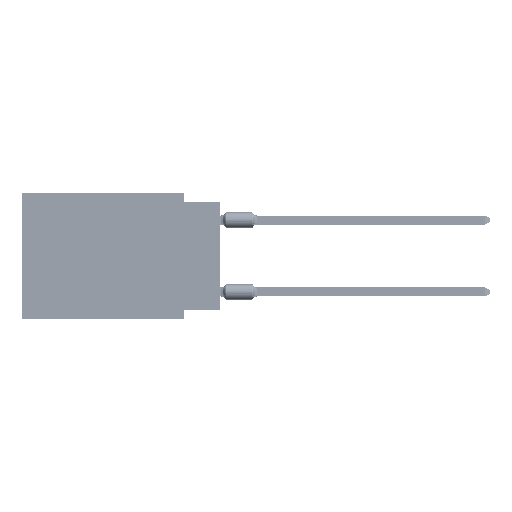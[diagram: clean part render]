
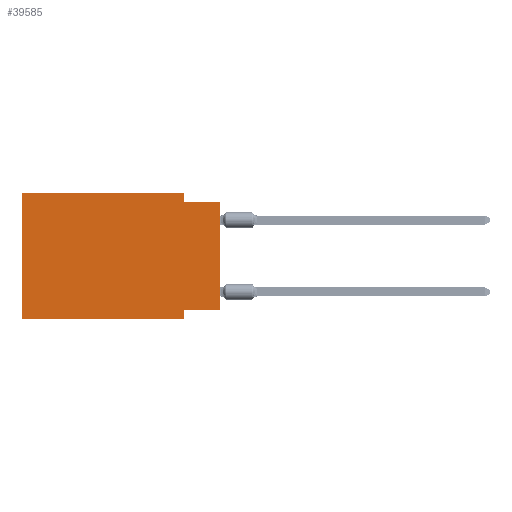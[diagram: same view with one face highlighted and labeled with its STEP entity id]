
A CAD part, left-side view. The second image highlights one B-rep face of the part: STEP entity #39585.
In plain terms, the highlighted planar face has unit normal (-1, 0, 0).
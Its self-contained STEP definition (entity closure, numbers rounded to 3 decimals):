
#471 = DIRECTION ( 'NONE',  ( 0., 0., -1. ) ) ;
#1553 = CARTESIAN_POINT ( 'NONE',  ( 0., 2.54, -8.255 ) ) ;
#2929 = EDGE_CURVE ( 'NONE', #44867, #82245, #107973, .T. ) ;
#6855 = LINE ( 'NONE', #51619, #43637 ) ;
#7664 = CARTESIAN_POINT ( 'NONE',  ( 0., 13.97, -8.89 ) ) ;
#10004 = VECTOR ( 'NONE', #471, 1000. ) ;
#10639 = DIRECTION ( 'NONE',  ( 0., 0., -1. ) ) ;
#10737 = EDGE_LOOP ( 'NONE', ( #77970, #42111, #17066, #55393, #105549, #76136, #22243, #19963 ) ) ;
#13198 = EDGE_CURVE ( 'NONE', #44867, #31810, #33668, .T. ) ;
#14741 = VECTOR ( 'NONE', #26188, 1000. ) ;
#14808 = VERTEX_POINT ( 'NONE', #32982 ) ;
#16562 = EDGE_CURVE ( 'NONE', #79509, #60646, #83438, .T. ) ;
#17066 = ORIENTED_EDGE ( 'NONE', *, *, #102104, .F. ) ;
#19963 = ORIENTED_EDGE ( 'NONE', *, *, #13198, .F. ) ;
#22243 = ORIENTED_EDGE ( 'NONE', *, *, #87698, .F. ) ;
#26188 = DIRECTION ( 'NONE',  ( 0., -1., 0. ) ) ;
#30516 = VECTOR ( 'NONE', #43050, 1000. ) ;
#31810 = VERTEX_POINT ( 'NONE', #1553 ) ;
#32205 = CARTESIAN_POINT ( 'NONE',  ( 0., 0., 0. ) ) ;
#32610 = VERTEX_POINT ( 'NONE', #76518 ) ;
#32982 = CARTESIAN_POINT ( 'NONE',  ( 0., 13.97, 0. ) ) ;
#33668 = LINE ( 'NONE', #85099, #30516 ) ;
#39585 = ADVANCED_FACE ( 'NONE', ( #55048 ), #72182, .F. ) ;
#41398 = DIRECTION ( 'NONE',  ( 0., -1., 0. ) ) ;
#42111 = ORIENTED_EDGE ( 'NONE', *, *, #86768, .F. ) ;
#43050 = DIRECTION ( 'NONE',  ( 0., 1., 0. ) ) ;
#43575 = CARTESIAN_POINT ( 'NONE',  ( 0., 2.54, -8.89 ) ) ;
#43637 = VECTOR ( 'NONE', #84829, 1000. ) ;
#44867 = VERTEX_POINT ( 'NONE', #65329 ) ;
#51619 = CARTESIAN_POINT ( 'NONE',  ( 0., 0., -0.635 ) ) ;
#54789 = VERTEX_POINT ( 'NONE', #64072 ) ;
#55048 = FACE_OUTER_BOUND ( 'NONE', #10737, .T. ) ;
#55305 = VECTOR ( 'NONE', #57617, 1000. ) ;
#55393 = ORIENTED_EDGE ( 'NONE', *, *, #65515, .F. ) ;
#57617 = DIRECTION ( 'NONE',  ( 0., 0., 1. ) ) ;
#60206 = LINE ( 'NONE', #43575, #10004 ) ;
#60646 = VERTEX_POINT ( 'NONE', #80372 ) ;
#60956 = LINE ( 'NONE', #86405, #72630 ) ;
#62259 = DIRECTION ( 'NONE',  ( 1., 0., 0. ) ) ;
#63890 = CARTESIAN_POINT ( 'NONE',  ( 0., 13.97, 0. ) ) ;
#64072 = CARTESIAN_POINT ( 'NONE',  ( 0., 2.54, 0. ) ) ;
#65329 = CARTESIAN_POINT ( 'NONE',  ( 0., 0., -8.255 ) ) ;
#65515 = EDGE_CURVE ( 'NONE', #14808, #54789, #86453, .T. ) ;
#67099 = VECTOR ( 'NONE', #104514, 1000. ) ;
#72182 = PLANE ( 'NONE',  #108007 ) ;
#72630 = VECTOR ( 'NONE', #10639, 1000. ) ;
#76136 = ORIENTED_EDGE ( 'NONE', *, *, #16562, .T. ) ;
#76518 = CARTESIAN_POINT ( 'NONE',  ( 0., 2.54, -0.635 ) ) ;
#77970 = ORIENTED_EDGE ( 'NONE', *, *, #2929, .T. ) ;
#79509 = VERTEX_POINT ( 'NONE', #90200 ) ;
#80372 = CARTESIAN_POINT ( 'NONE',  ( 0., 2.54, -8.89 ) ) ;
#82245 = VERTEX_POINT ( 'NONE', #107384 ) ;
#83438 = LINE ( 'NONE', #7664, #91496 ) ;
#84829 = DIRECTION ( 'NONE',  ( 0., -1., 0. ) ) ;
#85099 = CARTESIAN_POINT ( 'NONE',  ( 0., 0., -8.255 ) ) ;
#85898 = CARTESIAN_POINT ( 'NONE',  ( 0., 13.97, 0. ) ) ;
#86405 = CARTESIAN_POINT ( 'NONE',  ( 0., 2.54, 0. ) ) ;
#86453 = LINE ( 'NONE', #85898, #14741 ) ;
#86768 = EDGE_CURVE ( 'NONE', #32610, #82245, #6855, .T. ) ;
#87698 = EDGE_CURVE ( 'NONE', #31810, #60646, #60206, .T. ) ;
#89306 = DIRECTION ( 'NONE',  ( 0., 0., -1. ) ) ;
#90200 = CARTESIAN_POINT ( 'NONE',  ( 0., 13.97, -8.89 ) ) ;
#91496 = VECTOR ( 'NONE', #41398, 1000. ) ;
#95670 = LINE ( 'NONE', #102313, #67099 ) ;
#102104 = EDGE_CURVE ( 'NONE', #54789, #32610, #60956, .T. ) ;
#102313 = CARTESIAN_POINT ( 'NONE',  ( 0., 13.97, 0. ) ) ;
#102429 = EDGE_CURVE ( 'NONE', #79509, #14808, #95670, .T. ) ;
#104514 = DIRECTION ( 'NONE',  ( 0., 0., 1. ) ) ;
#105549 = ORIENTED_EDGE ( 'NONE', *, *, #102429, .F. ) ;
#107384 = CARTESIAN_POINT ( 'NONE',  ( 0., 0., -0.635 ) ) ;
#107973 = LINE ( 'NONE', #32205, #55305 ) ;
#108007 = AXIS2_PLACEMENT_3D ( 'NONE', #63890, #62259, #89306 ) ;
